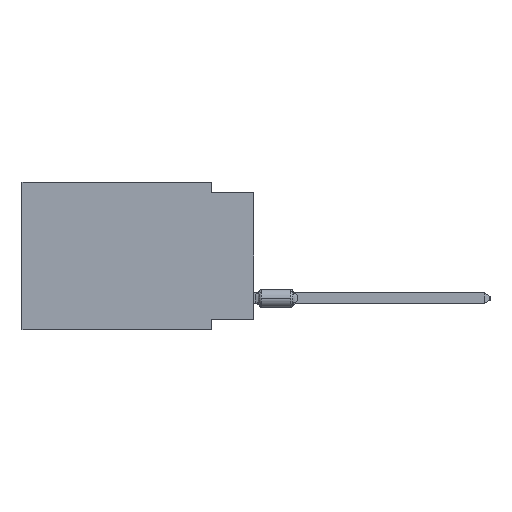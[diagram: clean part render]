
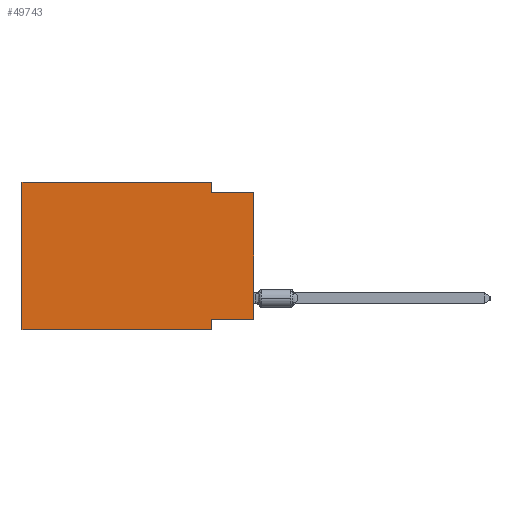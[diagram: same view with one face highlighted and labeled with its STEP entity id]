
A CAD part, left-side view. The second image highlights one B-rep face of the part: STEP entity #49743.
In plain terms, the highlighted planar face has unit normal (-1, 0, 0).
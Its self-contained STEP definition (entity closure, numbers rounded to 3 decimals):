
#590 = DIRECTION ( 'NONE',  ( 0., -1., 0. ) ) ;
#827 = EDGE_LOOP ( 'NONE', ( #60957, #57179, #3270, #48062, #21167, #56540, #83693, #66301 ) ) ;
#2484 = CARTESIAN_POINT ( 'NONE',  ( 0., 13.97, 0. ) ) ;
#2723 = DIRECTION ( 'NONE',  ( 0., 0., -1. ) ) ;
#3270 = ORIENTED_EDGE ( 'NONE', *, *, #87051, .F. ) ;
#4233 = CARTESIAN_POINT ( 'NONE',  ( 0., 0., -0.635 ) ) ;
#5450 = CARTESIAN_POINT ( 'NONE',  ( 0., 2.54, -8.89 ) ) ;
#6607 = LINE ( 'NONE', #7057, #72323 ) ;
#7057 = CARTESIAN_POINT ( 'NONE',  ( 0., 13.97, 0. ) ) ;
#9190 = CARTESIAN_POINT ( 'NONE',  ( 0., 13.97, 0. ) ) ;
#13213 = LINE ( 'NONE', #60486, #34765 ) ;
#13539 = DIRECTION ( 'NONE',  ( 0., 0., 1. ) ) ;
#14431 = CARTESIAN_POINT ( 'NONE',  ( 0., 0., 0. ) ) ;
#15734 = VERTEX_POINT ( 'NONE', #27817 ) ;
#17450 = VECTOR ( 'NONE', #13539, 1000. ) ;
#17847 = EDGE_CURVE ( 'NONE', #52423, #76959, #13213, .T. ) ;
#20727 = LINE ( 'NONE', #14431, #17450 ) ;
#21167 = ORIENTED_EDGE ( 'NONE', *, *, #77211, .F. ) ;
#23153 = DIRECTION ( 'NONE',  ( 1., 0., 0. ) ) ;
#23591 = DIRECTION ( 'NONE',  ( 0., 0., -1. ) ) ;
#25601 = CARTESIAN_POINT ( 'NONE',  ( 0., 0., -8.255 ) ) ;
#26113 = DIRECTION ( 'NONE',  ( 0., 0., -1. ) ) ;
#27817 = CARTESIAN_POINT ( 'NONE',  ( 0., 2.54, 0. ) ) ;
#29394 = LINE ( 'NONE', #9190, #75362 ) ;
#29524 = CARTESIAN_POINT ( 'NONE',  ( 0., 2.54, -8.255 ) ) ;
#30207 = VERTEX_POINT ( 'NONE', #84563 ) ;
#34765 = VECTOR ( 'NONE', #590, 1000. ) ;
#36470 = CARTESIAN_POINT ( 'NONE',  ( 0., 2.54, 0. ) ) ;
#36493 = EDGE_CURVE ( 'NONE', #42722, #15734, #6607, .T. ) ;
#36909 = LINE ( 'NONE', #36470, #67146 ) ;
#39695 = VERTEX_POINT ( 'NONE', #25601 ) ;
#40958 = EDGE_CURVE ( 'NONE', #39695, #72641, #41217, .T. ) ;
#41217 = LINE ( 'NONE', #56070, #74134 ) ;
#42722 = VERTEX_POINT ( 'NONE', #48496 ) ;
#44282 = EDGE_CURVE ( 'NONE', #51879, #30207, #78506, .T. ) ;
#44891 = EDGE_CURVE ( 'NONE', #39695, #30207, #20727, .T. ) ;
#45159 = DIRECTION ( 'NONE',  ( 0., -1., 0. ) ) ;
#47465 = CARTESIAN_POINT ( 'NONE',  ( 0., 2.54, -8.89 ) ) ;
#48062 = ORIENTED_EDGE ( 'NONE', *, *, #36493, .F. ) ;
#48496 = CARTESIAN_POINT ( 'NONE',  ( 0., 13.97, 0. ) ) ;
#49743 = ADVANCED_FACE ( 'NONE', ( #72203 ), #64565, .F. ) ;
#50116 = VECTOR ( 'NONE', #26113, 1000. ) ;
#51879 = VERTEX_POINT ( 'NONE', #65675 ) ;
#52423 = VERTEX_POINT ( 'NONE', #63896 ) ;
#55002 = EDGE_CURVE ( 'NONE', #72641, #76959, #67098, .T. ) ;
#56070 = CARTESIAN_POINT ( 'NONE',  ( 0., 0., -8.255 ) ) ;
#56540 = ORIENTED_EDGE ( 'NONE', *, *, #17847, .T. ) ;
#56669 = AXIS2_PLACEMENT_3D ( 'NONE', #2484, #23153, #23591 ) ;
#57179 = ORIENTED_EDGE ( 'NONE', *, *, #44282, .F. ) ;
#60486 = CARTESIAN_POINT ( 'NONE',  ( 0., 13.97, -8.89 ) ) ;
#60957 = ORIENTED_EDGE ( 'NONE', *, *, #44891, .T. ) ;
#63896 = CARTESIAN_POINT ( 'NONE',  ( 0., 13.97, -8.89 ) ) ;
#64565 = PLANE ( 'NONE',  #56669 ) ;
#65675 = CARTESIAN_POINT ( 'NONE',  ( 0., 2.54, -0.635 ) ) ;
#66301 = ORIENTED_EDGE ( 'NONE', *, *, #40958, .F. ) ;
#67098 = LINE ( 'NONE', #5450, #50116 ) ;
#67146 = VECTOR ( 'NONE', #2723, 1000. ) ;
#70024 = DIRECTION ( 'NONE',  ( 0., 1., 0. ) ) ;
#70822 = DIRECTION ( 'NONE',  ( 0., 0., 1. ) ) ;
#72203 = FACE_OUTER_BOUND ( 'NONE', #827, .T. ) ;
#72323 = VECTOR ( 'NONE', #80859, 1000. ) ;
#72641 = VERTEX_POINT ( 'NONE', #29524 ) ;
#74134 = VECTOR ( 'NONE', #70024, 1000. ) ;
#75362 = VECTOR ( 'NONE', #70822, 1000. ) ;
#76959 = VERTEX_POINT ( 'NONE', #47465 ) ;
#77211 = EDGE_CURVE ( 'NONE', #52423, #42722, #29394, .T. ) ;
#77360 = VECTOR ( 'NONE', #45159, 1000. ) ;
#78506 = LINE ( 'NONE', #4233, #77360 ) ;
#80859 = DIRECTION ( 'NONE',  ( 0., -1., 0. ) ) ;
#83693 = ORIENTED_EDGE ( 'NONE', *, *, #55002, .F. ) ;
#84563 = CARTESIAN_POINT ( 'NONE',  ( 0., 0., -0.635 ) ) ;
#87051 = EDGE_CURVE ( 'NONE', #15734, #51879, #36909, .T. ) ;
